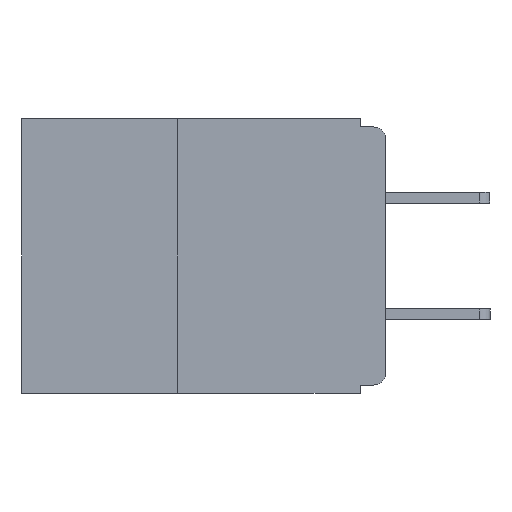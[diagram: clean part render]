
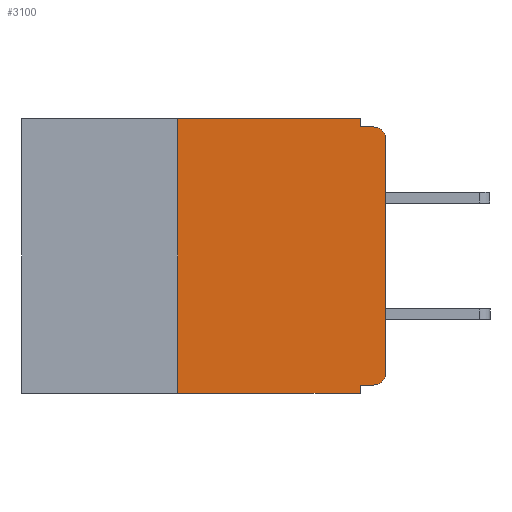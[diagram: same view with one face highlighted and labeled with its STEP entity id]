
A CAD part, left-side view. The second image highlights one B-rep face of the part: STEP entity #3100.
In plain terms, the highlighted planar face has unit normal (-1, 0, 0).
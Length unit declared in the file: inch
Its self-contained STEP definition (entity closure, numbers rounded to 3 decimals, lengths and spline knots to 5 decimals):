
#116 = CARTESIAN_POINT ( 'NONE',  ( 0., 0.031, 0. ) ) ;
#216 = ORIENTED_EDGE ( 'NONE', *, *, #5703, .T. ) ;
#270 = FACE_OUTER_BOUND ( 'NONE', #1412, .T. ) ;
#490 = ORIENTED_EDGE ( 'NONE', *, *, #4481, .F. ) ;
#694 = CARTESIAN_POINT ( 'NONE',  ( 0., 0.25, 0. ) ) ;
#1074 = CIRCLE ( 'NONE', #3270, 0.015 ) ;
#1113 = AXIS2_PLACEMENT_3D ( 'NONE', #9887, #11065, #11025 ) ;
#1366 = DIRECTION ( 'NONE',  ( 0., 0., -1. ) ) ;
#1412 = EDGE_LOOP ( 'NONE', ( #4589, #4273, #11132, #10311, #9822, #490, #216, #1727, #5007, #4980 ) ) ;
#1454 = CARTESIAN_POINT ( 'NONE',  ( 0., 0., 0. ) ) ;
#1588 = VECTOR ( 'NONE', #4726, 39.37008 ) ;
#1727 = ORIENTED_EDGE ( 'NONE', *, *, #11634, .F. ) ;
#1822 = LINE ( 'NONE', #4355, #1588 ) ;
#1851 = VERTEX_POINT ( 'NONE', #11238 ) ;
#1885 = EDGE_CURVE ( 'NONE', #7897, #4920, #10526, .T. ) ;
#2227 = AXIS2_PLACEMENT_3D ( 'NONE', #6208, #6279, #6094 ) ;
#2324 = EDGE_CURVE ( 'NONE', #3179, #8302, #1074, .T. ) ;
#2573 = EDGE_CURVE ( 'NONE', #4065, #8302, #3346, .T. ) ;
#3100 = ADVANCED_FACE ( 'NONE', ( #270 ), #11845, .F. ) ;
#3179 = VERTEX_POINT ( 'NONE', #9220 ) ;
#3270 = AXIS2_PLACEMENT_3D ( 'NONE', #7467, #11278, #1366 ) ;
#3346 = LINE ( 'NONE', #9612, #3955 ) ;
#3955 = VECTOR ( 'NONE', #6875, 39.37008 ) ;
#4065 = VERTEX_POINT ( 'NONE', #11167 ) ;
#4071 = EDGE_CURVE ( 'NONE', #4920, #4065, #9790, .T. ) ;
#4149 = VERTEX_POINT ( 'NONE', #7784 ) ;
#4273 = ORIENTED_EDGE ( 'NONE', *, *, #2324, .T. ) ;
#4355 = CARTESIAN_POINT ( 'NONE',  ( 0., 0.25, -0.33 ) ) ;
#4481 = EDGE_CURVE ( 'NONE', #7448, #7897, #1822, .T. ) ;
#4589 = ORIENTED_EDGE ( 'NONE', *, *, #7258, .T. ) ;
#4726 = DIRECTION ( 'NONE',  ( 0., 0., 1. ) ) ;
#4920 = VERTEX_POINT ( 'NONE', #11673 ) ;
#4980 = ORIENTED_EDGE ( 'NONE', *, *, #12072, .T. ) ;
#5007 = ORIENTED_EDGE ( 'NONE', *, *, #10398, .F. ) ;
#5469 = VECTOR ( 'NONE', #10830, 39.37008 ) ;
#5593 = DIRECTION ( 'NONE',  ( 0., 0., -1. ) ) ;
#5642 = CARTESIAN_POINT ( 'NONE',  ( 0., 0.031, -0.33 ) ) ;
#5703 = EDGE_CURVE ( 'NONE', #7448, #6005, #10208, .T. ) ;
#5936 = LINE ( 'NONE', #1454, #5976 ) ;
#5976 = VECTOR ( 'NONE', #11955, 39.37008 ) ;
#6005 = VERTEX_POINT ( 'NONE', #11208 ) ;
#6094 = DIRECTION ( 'NONE',  ( 0., 0., -1. ) ) ;
#6208 = CARTESIAN_POINT ( 'NONE',  ( 0., 0.015, -0.305 ) ) ;
#6279 = DIRECTION ( 'NONE',  ( -1., 0., 0. ) ) ;
#6585 = CARTESIAN_POINT ( 'NONE',  ( 0., 0.015, -0.01 ) ) ;
#6875 = DIRECTION ( 'NONE',  ( 0., -1., 0. ) ) ;
#7121 = VERTEX_POINT ( 'NONE', #10799 ) ;
#7258 = EDGE_CURVE ( 'NONE', #4149, #3179, #5936, .T. ) ;
#7448 = VERTEX_POINT ( 'NONE', #8055 ) ;
#7467 = CARTESIAN_POINT ( 'NONE',  ( 0., 0.015, -0.025 ) ) ;
#7784 = CARTESIAN_POINT ( 'NONE',  ( 0., 0., -0.305 ) ) ;
#7897 = VERTEX_POINT ( 'NONE', #694 ) ;
#8055 = CARTESIAN_POINT ( 'NONE',  ( 0., 0.25, -0.33 ) ) ;
#8174 = DIRECTION ( 'NONE',  ( 0., -1., 0. ) ) ;
#8218 = CARTESIAN_POINT ( 'NONE',  ( 0., 0.437, 0. ) ) ;
#8302 = VERTEX_POINT ( 'NONE', #6585 ) ;
#8358 = CARTESIAN_POINT ( 'NONE',  ( 0., 0.437, -0.33 ) ) ;
#9076 = CIRCLE ( 'NONE', #2227, 0.015 ) ;
#9220 = CARTESIAN_POINT ( 'NONE',  ( 0., 0., -0.025 ) ) ;
#9612 = CARTESIAN_POINT ( 'NONE',  ( 0., 0., -0.01 ) ) ;
#9790 = LINE ( 'NONE', #116, #5469 ) ;
#9822 = ORIENTED_EDGE ( 'NONE', *, *, #1885, .F. ) ;
#9836 = VECTOR ( 'NONE', #10365, 39.37008 ) ;
#9887 = CARTESIAN_POINT ( 'NONE',  ( 0., 0.437, 0. ) ) ;
#9955 = VECTOR ( 'NONE', #5593, 39.37008 ) ;
#9982 = LINE ( 'NONE', #5642, #9955 ) ;
#10208 = LINE ( 'NONE', #8358, #10235 ) ;
#10235 = VECTOR ( 'NONE', #8174, 39.37008 ) ;
#10311 = ORIENTED_EDGE ( 'NONE', *, *, #4071, .F. ) ;
#10365 = DIRECTION ( 'NONE',  ( 0., -1., 0. ) ) ;
#10398 = EDGE_CURVE ( 'NONE', #1851, #7121, #11841, .T. ) ;
#10526 = LINE ( 'NONE', #8218, #9836 ) ;
#10799 = CARTESIAN_POINT ( 'NONE',  ( 0., 0.031, -0.32 ) ) ;
#10830 = DIRECTION ( 'NONE',  ( 0., 0., -1. ) ) ;
#10965 = CARTESIAN_POINT ( 'NONE',  ( 0., 0., -0.32 ) ) ;
#11025 = DIRECTION ( 'NONE',  ( 0., 0., -1. ) ) ;
#11065 = DIRECTION ( 'NONE',  ( 1., 0., 0. ) ) ;
#11132 = ORIENTED_EDGE ( 'NONE', *, *, #2573, .F. ) ;
#11167 = CARTESIAN_POINT ( 'NONE',  ( 0., 0.031, -0.01 ) ) ;
#11208 = CARTESIAN_POINT ( 'NONE',  ( 0., 0.031, -0.33 ) ) ;
#11238 = CARTESIAN_POINT ( 'NONE',  ( 0., 0.015, -0.32 ) ) ;
#11278 = DIRECTION ( 'NONE',  ( -1., 0., 0. ) ) ;
#11362 = DIRECTION ( 'NONE',  ( 0., 1., 0. ) ) ;
#11634 = EDGE_CURVE ( 'NONE', #7121, #6005, #9982, .T. ) ;
#11673 = CARTESIAN_POINT ( 'NONE',  ( 0., 0.031, 0. ) ) ;
#11802 = VECTOR ( 'NONE', #11362, 39.37008 ) ;
#11841 = LINE ( 'NONE', #10965, #11802 ) ;
#11845 = PLANE ( 'NONE',  #1113 ) ;
#11955 = DIRECTION ( 'NONE',  ( 0., 0., 1. ) ) ;
#12072 = EDGE_CURVE ( 'NONE', #1851, #4149, #9076, .T. ) ;
